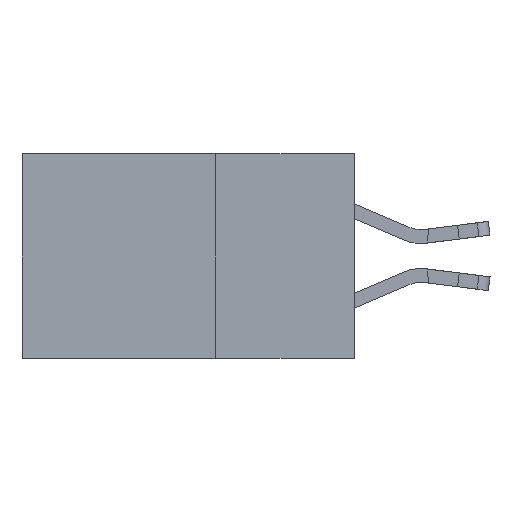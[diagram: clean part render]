
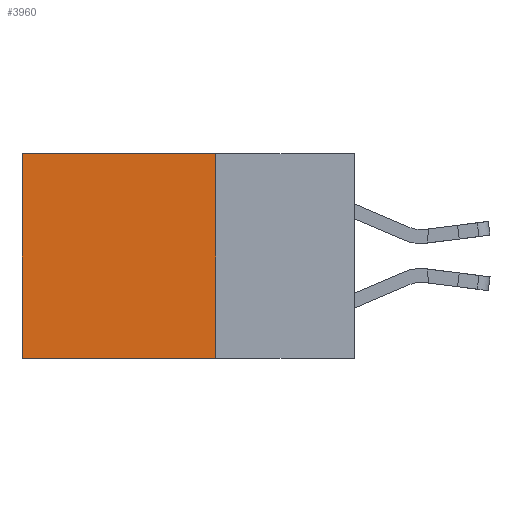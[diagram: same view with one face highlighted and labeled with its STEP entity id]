
A CAD part, left-side view. The second image highlights one B-rep face of the part: STEP entity #3960.
In plain terms, the highlighted planar face has unit normal (-1, 0, 0).
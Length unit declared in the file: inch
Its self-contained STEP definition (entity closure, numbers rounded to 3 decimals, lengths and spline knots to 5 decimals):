
#425 = VERTEX_POINT ( 'NONE', #1465 ) ;
#551 = EDGE_LOOP ( 'NONE', ( #5258, #1149, #19867, #5487 ) ) ;
#623 = LINE ( 'NONE', #3504, #8933 ) ;
#1149 = ORIENTED_EDGE ( 'NONE', *, *, #4377, .F. ) ;
#1403 = VECTOR ( 'NONE', #16747, 39.37008 ) ;
#1465 = CARTESIAN_POINT ( 'NONE',  ( 0.2615, 0.6, -0.37 ) ) ;
#3504 = CARTESIAN_POINT ( 'NONE',  ( 0.2615, 0.25, 0. ) ) ;
#3960 = ADVANCED_FACE ( 'NONE', ( #17462 ), #10597, .F. ) ;
#4377 = EDGE_CURVE ( 'NONE', #18920, #425, #14125, .T. ) ;
#4508 = CARTESIAN_POINT ( 'NONE',  ( 0.2615, 0.6, -0.37 ) ) ;
#5099 = VERTEX_POINT ( 'NONE', #7338 ) ;
#5258 = ORIENTED_EDGE ( 'NONE', *, *, #19526, .T. ) ;
#5487 = ORIENTED_EDGE ( 'NONE', *, *, #18978, .T. ) ;
#6180 = DIRECTION ( 'NONE',  ( 0., 0., -1. ) ) ;
#7338 = CARTESIAN_POINT ( 'NONE',  ( 0.2615, 0.25, 0. ) ) ;
#8933 = VECTOR ( 'NONE', #10031, 39.37008 ) ;
#10031 = DIRECTION ( 'NONE',  ( 0., 1., 0. ) ) ;
#10162 = DIRECTION ( 'NONE',  ( 0., 0., -1. ) ) ;
#10181 = DIRECTION ( 'NONE',  ( 1., 0., 0. ) ) ;
#10186 = LINE ( 'NONE', #11819, #1403 ) ;
#10240 = VERTEX_POINT ( 'NONE', #14169 ) ;
#10492 = CARTESIAN_POINT ( 'NONE',  ( 0.2615, 0.25, -0.37 ) ) ;
#10597 = PLANE ( 'NONE',  #12013 ) ;
#11701 = LINE ( 'NONE', #4508, #20830 ) ;
#11819 = CARTESIAN_POINT ( 'NONE',  ( 0.2615, 0.25, -0.37 ) ) ;
#12013 = AXIS2_PLACEMENT_3D ( 'NONE', #10492, #10181, #10162 ) ;
#14125 = LINE ( 'NONE', #19126, #17443 ) ;
#14169 = CARTESIAN_POINT ( 'NONE',  ( 0.2615, 0.6, 0. ) ) ;
#14881 = CARTESIAN_POINT ( 'NONE',  ( 0.2615, 0.25, -0.37 ) ) ;
#16747 = DIRECTION ( 'NONE',  ( 0., 0., -1. ) ) ;
#17443 = VECTOR ( 'NONE', #18984, 39.37008 ) ;
#17462 = FACE_OUTER_BOUND ( 'NONE', #551, .T. ) ;
#18920 = VERTEX_POINT ( 'NONE', #14881 ) ;
#18978 = EDGE_CURVE ( 'NONE', #5099, #10240, #623, .T. ) ;
#18984 = DIRECTION ( 'NONE',  ( 0., 1., 0. ) ) ;
#19126 = CARTESIAN_POINT ( 'NONE',  ( 0.2615, 0.25, -0.37 ) ) ;
#19177 = EDGE_CURVE ( 'NONE', #5099, #18920, #10186, .T. ) ;
#19526 = EDGE_CURVE ( 'NONE', #10240, #425, #11701, .T. ) ;
#19867 = ORIENTED_EDGE ( 'NONE', *, *, #19177, .F. ) ;
#20830 = VECTOR ( 'NONE', #6180, 39.37008 ) ;
